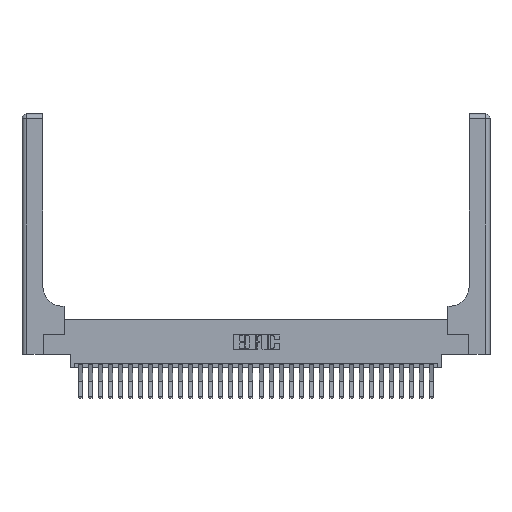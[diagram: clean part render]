
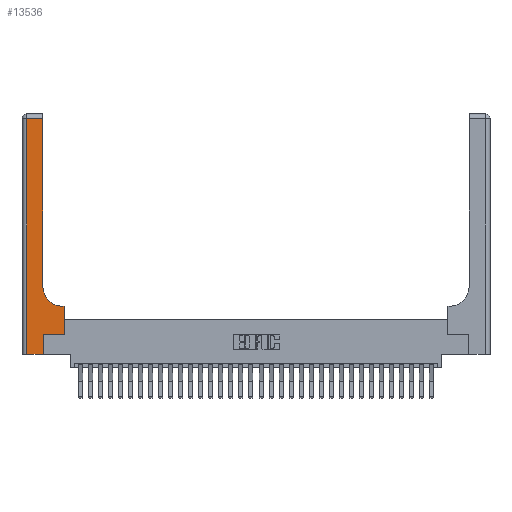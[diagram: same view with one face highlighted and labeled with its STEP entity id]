
A CAD part, top view. The second image highlights one B-rep face of the part: STEP entity #13536.
In plain terms, the highlighted planar face has unit normal (0, 0, 1).
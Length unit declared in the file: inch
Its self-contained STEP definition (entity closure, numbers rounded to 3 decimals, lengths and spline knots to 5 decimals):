
#345 = AXIS2_PLACEMENT_3D ( 'NONE', #6729, #21376, #25370 ) ;
#556 = EDGE_CURVE ( 'NONE', #8228, #13796, #15339, .T. ) ;
#1712 = VECTOR ( 'NONE', #16561, 39.37008 ) ;
#1979 = CARTESIAN_POINT ( 'NONE',  ( 0.528, 0.6, 0.37 ) ) ;
#2937 = CARTESIAN_POINT ( 'NONE',  ( 0.06, 2.94, 0.37 ) ) ;
#3423 = CARTESIAN_POINT ( 'NONE',  ( 0.26, 3., 0.37 ) ) ;
#3751 = DIRECTION ( 'NONE',  ( 0., 1., 0. ) ) ;
#3875 = DIRECTION ( 'NONE',  ( 0., 0., -1. ) ) ;
#4145 = EDGE_CURVE ( 'NONE', #20065, #22911, #8998, .T. ) ;
#4183 = CARTESIAN_POINT ( 'NONE',  ( 0.51, 0.85, 0.37 ) ) ;
#4610 = PLANE ( 'NONE',  #345 ) ;
#4641 = LINE ( 'NONE', #25857, #21234 ) ;
#5048 = FACE_OUTER_BOUND ( 'NONE', #26392, .T. ) ;
#5840 = ORIENTED_EDGE ( 'NONE', *, *, #4145, .T. ) ;
#5865 = VERTEX_POINT ( 'NONE', #13242 ) ;
#6312 = DIRECTION ( 'NONE',  ( -1., 0., 0. ) ) ;
#6315 = CARTESIAN_POINT ( 'NONE',  ( 0.528, 0.25, 0.37 ) ) ;
#6729 = CARTESIAN_POINT ( 'NONE',  ( 0., 3., 0.37 ) ) ;
#6832 = VERTEX_POINT ( 'NONE', #27658 ) ;
#6854 = VECTOR ( 'NONE', #28952, 39.37008 ) ;
#7606 = EDGE_CURVE ( 'NONE', #26105, #20065, #19932, .T. ) ;
#8228 = VERTEX_POINT ( 'NONE', #6315 ) ;
#8413 = ORIENTED_EDGE ( 'NONE', *, *, #7606, .T. ) ;
#8998 = LINE ( 'NONE', #20287, #25074 ) ;
#9636 = AXIS2_PLACEMENT_3D ( 'NONE', #4183, #3875, #24945 ) ;
#9896 = CARTESIAN_POINT ( 'NONE',  ( 0.265, 0.25, 0.37 ) ) ;
#11496 = EDGE_CURVE ( 'NONE', #22911, #5865, #28468, .T. ) ;
#11865 = EDGE_CURVE ( 'NONE', #5865, #19077, #4641, .T. ) ;
#13044 = VECTOR ( 'NONE', #24039, 39.37008 ) ;
#13242 = CARTESIAN_POINT ( 'NONE',  ( 0.265, 0., 0.37 ) ) ;
#13536 = ADVANCED_FACE ( 'NONE', ( #5048 ), #4610, .F. ) ;
#13796 = VERTEX_POINT ( 'NONE', #1979 ) ;
#14079 = EDGE_CURVE ( 'NONE', #13796, #20120, #29522, .T. ) ;
#14765 = EDGE_CURVE ( 'NONE', #20120, #6832, #25198, .T. ) ;
#15038 = ORIENTED_EDGE ( 'NONE', *, *, #14079, .T. ) ;
#15339 = LINE ( 'NONE', #24664, #22133 ) ;
#15436 = CARTESIAN_POINT ( 'NONE',  ( 0.51, 0.6, 0.37 ) ) ;
#16140 = DIRECTION ( 'NONE',  ( 1., 0., 0. ) ) ;
#16300 = EDGE_CURVE ( 'NONE', #6832, #26105, #28617, .T. ) ;
#16443 = CARTESIAN_POINT ( 'NONE',  ( 0.265, 0.25, 0.37 ) ) ;
#16561 = DIRECTION ( 'NONE',  ( 1., 0., 0. ) ) ;
#18844 = CARTESIAN_POINT ( 'NONE',  ( 0., 0., 0.37 ) ) ;
#19077 = VERTEX_POINT ( 'NONE', #9896 ) ;
#19521 = EDGE_CURVE ( 'NONE', #19077, #8228, #28052, .T. ) ;
#19637 = CARTESIAN_POINT ( 'NONE',  ( 0., 2.94, 0.37 ) ) ;
#19706 = CARTESIAN_POINT ( 'NONE',  ( 0.06, 0., 0.37 ) ) ;
#19932 = LINE ( 'NONE', #19637, #6854 ) ;
#20065 = VERTEX_POINT ( 'NONE', #2937 ) ;
#20120 = VERTEX_POINT ( 'NONE', #15436 ) ;
#20287 = CARTESIAN_POINT ( 'NONE',  ( 0.06, 3., 0.37 ) ) ;
#20440 = DIRECTION ( 'NONE',  ( 0., -1., 0. ) ) ;
#21234 = VECTOR ( 'NONE', #23399, 39.37008 ) ;
#21376 = DIRECTION ( 'NONE',  ( 0., 0., -1. ) ) ;
#22133 = VECTOR ( 'NONE', #3751, 39.37008 ) ;
#22805 = CARTESIAN_POINT ( 'NONE',  ( 0.26, 0.6, 0.37 ) ) ;
#22911 = VERTEX_POINT ( 'NONE', #19706 ) ;
#22988 = ORIENTED_EDGE ( 'NONE', *, *, #14765, .T. ) ;
#23399 = DIRECTION ( 'NONE',  ( 0., 1., 0. ) ) ;
#23942 = ORIENTED_EDGE ( 'NONE', *, *, #556, .T. ) ;
#24039 = DIRECTION ( 'NONE',  ( 0., 1., 0. ) ) ;
#24664 = CARTESIAN_POINT ( 'NONE',  ( 0.528, 0.25, 0.37 ) ) ;
#24945 = DIRECTION ( 'NONE',  ( 1., 0., 0. ) ) ;
#25074 = VECTOR ( 'NONE', #20440, 39.37008 ) ;
#25198 = CIRCLE ( 'NONE', #9636, 0.25 ) ;
#25370 = DIRECTION ( 'NONE',  ( -1., 0., 0. ) ) ;
#25857 = CARTESIAN_POINT ( 'NONE',  ( 0.265, 0., 0.37 ) ) ;
#26105 = VERTEX_POINT ( 'NONE', #29809 ) ;
#26392 = EDGE_LOOP ( 'NONE', ( #28671, #8413, #5840, #29869, #28113, #27875, #23942, #15038, #22988 ) ) ;
#26687 = VECTOR ( 'NONE', #6312, 39.37008 ) ;
#26811 = VECTOR ( 'NONE', #16140, 39.37008 ) ;
#27658 = CARTESIAN_POINT ( 'NONE',  ( 0.26, 0.85, 0.37 ) ) ;
#27875 = ORIENTED_EDGE ( 'NONE', *, *, #19521, .T. ) ;
#28052 = LINE ( 'NONE', #16443, #26811 ) ;
#28113 = ORIENTED_EDGE ( 'NONE', *, *, #11865, .T. ) ;
#28468 = LINE ( 'NONE', #18844, #1712 ) ;
#28617 = LINE ( 'NONE', #3423, #13044 ) ;
#28671 = ORIENTED_EDGE ( 'NONE', *, *, #16300, .T. ) ;
#28952 = DIRECTION ( 'NONE',  ( -1., 0., 0. ) ) ;
#29522 = LINE ( 'NONE', #22805, #26687 ) ;
#29809 = CARTESIAN_POINT ( 'NONE',  ( 0.26, 2.94, 0.37 ) ) ;
#29869 = ORIENTED_EDGE ( 'NONE', *, *, #11496, .T. ) ;
